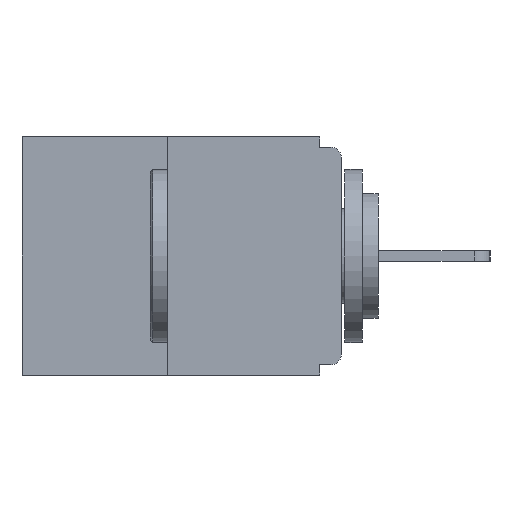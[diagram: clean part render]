
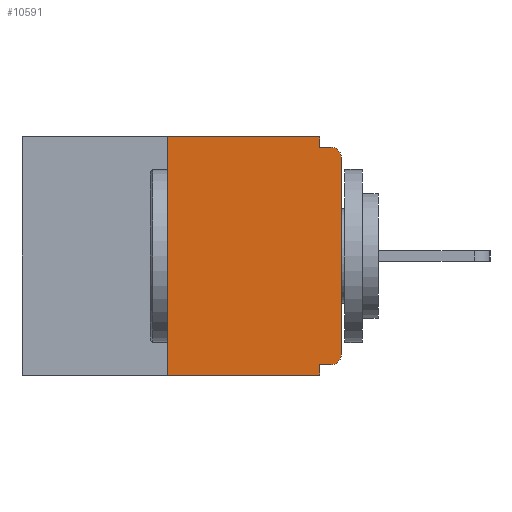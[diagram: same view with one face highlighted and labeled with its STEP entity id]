
A CAD part, left-side view. The second image highlights one B-rep face of the part: STEP entity #10591.
In plain terms, the highlighted planar face has unit normal (-1, 0, 0).
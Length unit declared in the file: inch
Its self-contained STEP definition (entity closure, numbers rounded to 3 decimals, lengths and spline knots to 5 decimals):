
#101 = DIRECTION ( 'NONE',  ( 1., 0., 0. ) ) ;
#268 = EDGE_CURVE ( 'NONE', #3644, #5814, #14897, .T. ) ;
#329 = VERTEX_POINT ( 'NONE', #813 ) ;
#337 = FACE_OUTER_BOUND ( 'NONE', #7342, .T. ) ;
#361 = VERTEX_POINT ( 'NONE', #10693 ) ;
#678 = DIRECTION ( 'NONE',  ( 0., 0., 1. ) ) ;
#813 = CARTESIAN_POINT ( 'NONE',  ( 0., 0.015, -0.328 ) ) ;
#821 = EDGE_CURVE ( 'NONE', #4090, #5814, #7212, .T. ) ;
#845 = DIRECTION ( 'NONE',  ( 0., 1., 0. ) ) ;
#1375 = CARTESIAN_POINT ( 'NONE',  ( 0., 0.015, -0.015 ) ) ;
#1494 = CARTESIAN_POINT ( 'NONE',  ( 0., 0.031, -0.015 ) ) ;
#1872 = EDGE_CURVE ( 'NONE', #3644, #13656, #6356, .T. ) ;
#2377 = ORIENTED_EDGE ( 'NONE', *, *, #10206, .F. ) ;
#2465 = VECTOR ( 'NONE', #6569, 39.37008 ) ;
#2754 = CARTESIAN_POINT ( 'NONE',  ( 0., 0.46, 0. ) ) ;
#2793 = VECTOR ( 'NONE', #13033, 39.37008 ) ;
#3644 = VERTEX_POINT ( 'NONE', #5797 ) ;
#3706 = VECTOR ( 'NONE', #7334, 39.37008 ) ;
#3713 = AXIS2_PLACEMENT_3D ( 'NONE', #12617, #7006, #11688 ) ;
#4090 = VERTEX_POINT ( 'NONE', #14673 ) ;
#4370 = ORIENTED_EDGE ( 'NONE', *, *, #7906, .F. ) ;
#4495 = CARTESIAN_POINT ( 'NONE',  ( 0., 0., -0.328 ) ) ;
#5250 = LINE ( 'NONE', #9857, #12397 ) ;
#5737 = EDGE_CURVE ( 'NONE', #10403, #7034, #6441, .T. ) ;
#5762 = VERTEX_POINT ( 'NONE', #10924 ) ;
#5797 = CARTESIAN_POINT ( 'NONE',  ( 0., 0.25, -0.343 ) ) ;
#5814 = VERTEX_POINT ( 'NONE', #11290 ) ;
#5877 = LINE ( 'NONE', #9276, #2793 ) ;
#5945 = ORIENTED_EDGE ( 'NONE', *, *, #1872, .F. ) ;
#6094 = DIRECTION ( 'NONE',  ( 0., 0., -1. ) ) ;
#6244 = CARTESIAN_POINT ( 'NONE',  ( 0., 0.015, -0.03 ) ) ;
#6356 = LINE ( 'NONE', #14927, #11597 ) ;
#6441 = CIRCLE ( 'NONE', #6926, 0.015 ) ;
#6569 = DIRECTION ( 'NONE',  ( 0., -1., 0. ) ) ;
#6926 = AXIS2_PLACEMENT_3D ( 'NONE', #6244, #9923, #13313 ) ;
#6972 = VECTOR ( 'NONE', #845, 39.37008 ) ;
#6997 = ORIENTED_EDGE ( 'NONE', *, *, #5737, .T. ) ;
#7006 = DIRECTION ( 'NONE',  ( -1., 0., 0. ) ) ;
#7034 = VERTEX_POINT ( 'NONE', #1375 ) ;
#7212 = LINE ( 'NONE', #8350, #13405 ) ;
#7334 = DIRECTION ( 'NONE',  ( 0., 0., -1. ) ) ;
#7342 = EDGE_LOOP ( 'NONE', ( #10785, #5945, #10914, #9229, #4370, #14223, #10013, #6997, #7869, #2377 ) ) ;
#7869 = ORIENTED_EDGE ( 'NONE', *, *, #10355, .F. ) ;
#7906 = EDGE_CURVE ( 'NONE', #329, #4090, #11428, .T. ) ;
#8135 = EDGE_CURVE ( 'NONE', #361, #10403, #5877, .T. ) ;
#8350 = CARTESIAN_POINT ( 'NONE',  ( 0., 0.031, -0.343 ) ) ;
#8664 = CARTESIAN_POINT ( 'NONE',  ( 0., 0.25, 0. ) ) ;
#8933 = CARTESIAN_POINT ( 'NONE',  ( 0., 0., -0.03 ) ) ;
#9003 = CARTESIAN_POINT ( 'NONE',  ( 0., 0.46, -0.343 ) ) ;
#9229 = ORIENTED_EDGE ( 'NONE', *, *, #821, .F. ) ;
#9276 = CARTESIAN_POINT ( 'NONE',  ( 0., 0., 0. ) ) ;
#9377 = VERTEX_POINT ( 'NONE', #1494 ) ;
#9857 = CARTESIAN_POINT ( 'NONE',  ( 0., 0.46, 0. ) ) ;
#9923 = DIRECTION ( 'NONE',  ( -1., 0., 0. ) ) ;
#9947 = DIRECTION ( 'NONE',  ( 0., -1., 0. ) ) ;
#10013 = ORIENTED_EDGE ( 'NONE', *, *, #8135, .T. ) ;
#10206 = EDGE_CURVE ( 'NONE', #5762, #9377, #13110, .T. ) ;
#10355 = EDGE_CURVE ( 'NONE', #9377, #7034, #11314, .T. ) ;
#10403 = VERTEX_POINT ( 'NONE', #8933 ) ;
#10591 = ADVANCED_FACE ( 'NONE', ( #337 ), #13248, .F. ) ;
#10693 = CARTESIAN_POINT ( 'NONE',  ( 0., 0., -0.313 ) ) ;
#10785 = ORIENTED_EDGE ( 'NONE', *, *, #14639, .F. ) ;
#10884 = EDGE_CURVE ( 'NONE', #329, #361, #11593, .T. ) ;
#10914 = ORIENTED_EDGE ( 'NONE', *, *, #268, .T. ) ;
#10924 = CARTESIAN_POINT ( 'NONE',  ( 0., 0.031, 0. ) ) ;
#11082 = AXIS2_PLACEMENT_3D ( 'NONE', #2754, #101, #6094 ) ;
#11290 = CARTESIAN_POINT ( 'NONE',  ( 0., 0.031, -0.343 ) ) ;
#11314 = LINE ( 'NONE', #13665, #2465 ) ;
#11428 = LINE ( 'NONE', #4495, #6972 ) ;
#11593 = CIRCLE ( 'NONE', #3713, 0.015 ) ;
#11594 = DIRECTION ( 'NONE',  ( 0., 0., -1. ) ) ;
#11597 = VECTOR ( 'NONE', #678, 39.37008 ) ;
#11688 = DIRECTION ( 'NONE',  ( 0., 0., -1. ) ) ;
#11950 = CARTESIAN_POINT ( 'NONE',  ( 0., 0.031, 0. ) ) ;
#12397 = VECTOR ( 'NONE', #9947, 39.37008 ) ;
#12617 = CARTESIAN_POINT ( 'NONE',  ( 0., 0.015, -0.313 ) ) ;
#12866 = VECTOR ( 'NONE', #15120, 39.37008 ) ;
#13033 = DIRECTION ( 'NONE',  ( 0., 0., 1. ) ) ;
#13110 = LINE ( 'NONE', #11950, #3706 ) ;
#13248 = PLANE ( 'NONE',  #11082 ) ;
#13313 = DIRECTION ( 'NONE',  ( 0., 0., -1. ) ) ;
#13405 = VECTOR ( 'NONE', #11594, 39.37008 ) ;
#13656 = VERTEX_POINT ( 'NONE', #8664 ) ;
#13665 = CARTESIAN_POINT ( 'NONE',  ( 0., 0., -0.015 ) ) ;
#14223 = ORIENTED_EDGE ( 'NONE', *, *, #10884, .T. ) ;
#14639 = EDGE_CURVE ( 'NONE', #13656, #5762, #5250, .T. ) ;
#14673 = CARTESIAN_POINT ( 'NONE',  ( 0., 0.031, -0.328 ) ) ;
#14897 = LINE ( 'NONE', #9003, #12866 ) ;
#14927 = CARTESIAN_POINT ( 'NONE',  ( 0., 0.25, 0. ) ) ;
#15120 = DIRECTION ( 'NONE',  ( 0., -1., 0. ) ) ;
